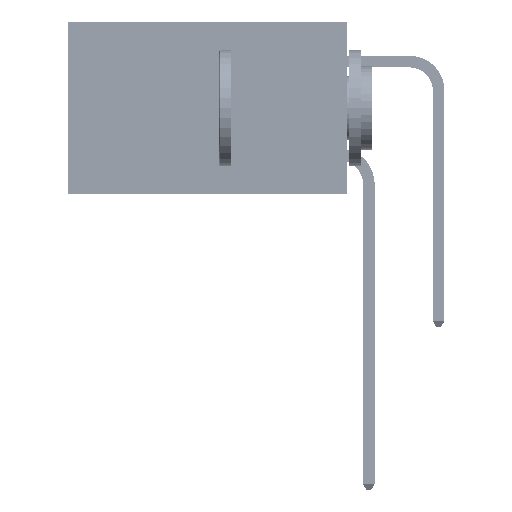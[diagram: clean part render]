
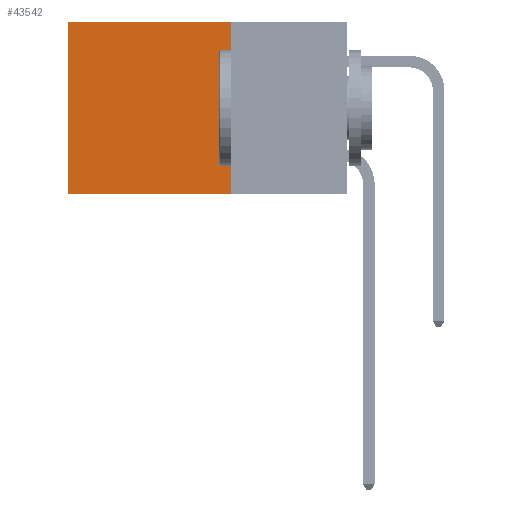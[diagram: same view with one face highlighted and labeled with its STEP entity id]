
A CAD part, left-side view. The second image highlights one B-rep face of the part: STEP entity #43542.
In plain terms, the highlighted planar face has unit normal (-1, 0, 0).
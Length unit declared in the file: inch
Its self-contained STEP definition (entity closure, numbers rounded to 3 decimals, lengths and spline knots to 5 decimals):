
#423 = DIRECTION ( 'NONE',  ( 0., 1., 0. ) ) ;
#2596 = VERTEX_POINT ( 'NONE', #4595 ) ;
#4595 = CARTESIAN_POINT ( 'NONE',  ( 0.2875, 0.25, 0. ) ) ;
#6390 = EDGE_CURVE ( 'NONE', #48022, #26710, #9201, .T. ) ;
#6509 = LINE ( 'NONE', #48642, #47354 ) ;
#6939 = PLANE ( 'NONE',  #8815 ) ;
#8711 = CARTESIAN_POINT ( 'NONE',  ( 0.2875, 0.25, 0. ) ) ;
#8815 = AXIS2_PLACEMENT_3D ( 'NONE', #31435, #43671, #19312 ) ;
#9201 = LINE ( 'NONE', #13456, #51289 ) ;
#10833 = LINE ( 'NONE', #13160, #51618 ) ;
#12106 = DIRECTION ( 'NONE',  ( 0., 0., -1. ) ) ;
#13160 = CARTESIAN_POINT ( 'NONE',  ( 0.2875, 0.6, 0. ) ) ;
#13456 = CARTESIAN_POINT ( 'NONE',  ( 0.2875, 0.25, -0.37 ) ) ;
#15960 = VECTOR ( 'NONE', #423, 39.37008 ) ;
#17599 = DIRECTION ( 'NONE',  ( 0., 1., 0. ) ) ;
#19312 = DIRECTION ( 'NONE',  ( 0., 0., -1. ) ) ;
#20499 = EDGE_CURVE ( 'NONE', #2596, #32644, #28083, .T. ) ;
#25117 = EDGE_CURVE ( 'NONE', #32644, #26710, #10833, .T. ) ;
#26710 = VERTEX_POINT ( 'NONE', #41937 ) ;
#28083 = LINE ( 'NONE', #8711, #15960 ) ;
#29499 = CARTESIAN_POINT ( 'NONE',  ( 0.2875, 0.6, 0. ) ) ;
#29558 = EDGE_LOOP ( 'NONE', ( #46278, #36166, #38621, #32053 ) ) ;
#31435 = CARTESIAN_POINT ( 'NONE',  ( 0.2875, 0.25, 0. ) ) ;
#32053 = ORIENTED_EDGE ( 'NONE', *, *, #20499, .T. ) ;
#32644 = VERTEX_POINT ( 'NONE', #29499 ) ;
#36166 = ORIENTED_EDGE ( 'NONE', *, *, #6390, .F. ) ;
#37608 = DIRECTION ( 'NONE',  ( 0., 0., -1. ) ) ;
#38621 = ORIENTED_EDGE ( 'NONE', *, *, #41758, .F. ) ;
#41758 = EDGE_CURVE ( 'NONE', #2596, #48022, #6509, .T. ) ;
#41937 = CARTESIAN_POINT ( 'NONE',  ( 0.2875, 0.6, -0.37 ) ) ;
#43542 = ADVANCED_FACE ( 'NONE', ( #50428 ), #6939, .F. ) ;
#43671 = DIRECTION ( 'NONE',  ( 1., 0., 0. ) ) ;
#46278 = ORIENTED_EDGE ( 'NONE', *, *, #25117, .T. ) ;
#47354 = VECTOR ( 'NONE', #12106, 39.37008 ) ;
#48022 = VERTEX_POINT ( 'NONE', #52159 ) ;
#48642 = CARTESIAN_POINT ( 'NONE',  ( 0.2875, 0.25, 0. ) ) ;
#50428 = FACE_OUTER_BOUND ( 'NONE', #29558, .T. ) ;
#51289 = VECTOR ( 'NONE', #17599, 39.37008 ) ;
#51618 = VECTOR ( 'NONE', #37608, 39.37008 ) ;
#52159 = CARTESIAN_POINT ( 'NONE',  ( 0.2875, 0.25, -0.37 ) ) ;
